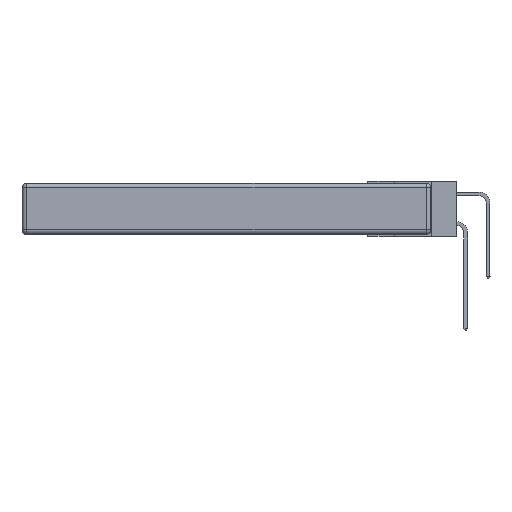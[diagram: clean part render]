
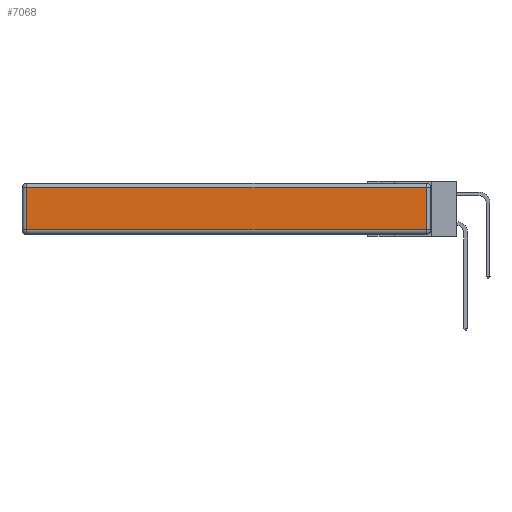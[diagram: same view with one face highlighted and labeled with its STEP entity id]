
A CAD part, left-side view. The second image highlights one B-rep face of the part: STEP entity #7068.
In plain terms, the highlighted planar face has unit normal (-1, 0, 0).
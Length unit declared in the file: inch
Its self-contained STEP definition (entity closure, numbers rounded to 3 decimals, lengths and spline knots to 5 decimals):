
#49 = DIRECTION ( 'NONE',  ( -1., 0., 0. ) ) ;
#170 = LINE ( 'NONE', #4414, #16548 ) ;
#312 = VECTOR ( 'NONE', #8222, 39.37008 ) ;
#349 = VERTEX_POINT ( 'NONE', #13392 ) ;
#1100 = ORIENTED_EDGE ( 'NONE', *, *, #12529, .T. ) ;
#2550 = LINE ( 'NONE', #3947, #312 ) ;
#2683 = PLANE ( 'NONE',  #12346 ) ;
#2708 = ORIENTED_EDGE ( 'NONE', *, *, #4282, .T. ) ;
#2982 = CARTESIAN_POINT ( 'NONE',  ( 0., 2.72, -0.03 ) ) ;
#3947 = CARTESIAN_POINT ( 'NONE',  ( 0., 0.03, -0.343 ) ) ;
#4282 = EDGE_CURVE ( 'NONE', #349, #6377, #13627, .T. ) ;
#4414 = CARTESIAN_POINT ( 'NONE',  ( 0., 0., -0.313 ) ) ;
#4867 = LINE ( 'NONE', #13425, #15159 ) ;
#6377 = VERTEX_POINT ( 'NONE', #2982 ) ;
#7068 = ADVANCED_FACE ( 'NONE', ( #7208 ), #2683, .T. ) ;
#7101 = VECTOR ( 'NONE', #7996, 39.37008 ) ;
#7208 = FACE_OUTER_BOUND ( 'NONE', #10451, .T. ) ;
#7384 = CARTESIAN_POINT ( 'NONE',  ( 0., 2.72, -0.313 ) ) ;
#7996 = DIRECTION ( 'NONE',  ( 0., 1., 0. ) ) ;
#8222 = DIRECTION ( 'NONE',  ( 0., 0., 1. ) ) ;
#8517 = DIRECTION ( 'NONE',  ( 0., 0., 1. ) ) ;
#9200 = CARTESIAN_POINT ( 'NONE',  ( 0., 0.03, -0.313 ) ) ;
#10451 = EDGE_LOOP ( 'NONE', ( #1100, #18213, #2708, #12137 ) ) ;
#10683 = DIRECTION ( 'NONE',  ( 0., 0., -1. ) ) ;
#12137 = ORIENTED_EDGE ( 'NONE', *, *, #12979, .T. ) ;
#12346 = AXIS2_PLACEMENT_3D ( 'NONE', #18437, #49, #8517 ) ;
#12529 = EDGE_CURVE ( 'NONE', #16921, #13520, #170, .T. ) ;
#12979 = EDGE_CURVE ( 'NONE', #6377, #16921, #4867, .T. ) ;
#13392 = CARTESIAN_POINT ( 'NONE',  ( 0., 0.03, -0.03 ) ) ;
#13425 = CARTESIAN_POINT ( 'NONE',  ( 0., 2.72, -0.343 ) ) ;
#13520 = VERTEX_POINT ( 'NONE', #9200 ) ;
#13627 = LINE ( 'NONE', #16584, #7101 ) ;
#14502 = DIRECTION ( 'NONE',  ( 0., -1., 0. ) ) ;
#14968 = EDGE_CURVE ( 'NONE', #13520, #349, #2550, .T. ) ;
#15159 = VECTOR ( 'NONE', #10683, 39.37008 ) ;
#16548 = VECTOR ( 'NONE', #14502, 39.37008 ) ;
#16584 = CARTESIAN_POINT ( 'NONE',  ( 0., 2.75, -0.03 ) ) ;
#16921 = VERTEX_POINT ( 'NONE', #7384 ) ;
#18213 = ORIENTED_EDGE ( 'NONE', *, *, #14968, .T. ) ;
#18437 = CARTESIAN_POINT ( 'NONE',  ( 0., 0., -0.343 ) ) ;
